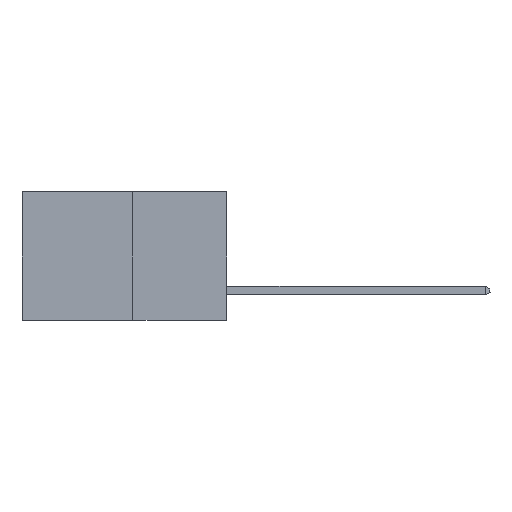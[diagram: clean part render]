
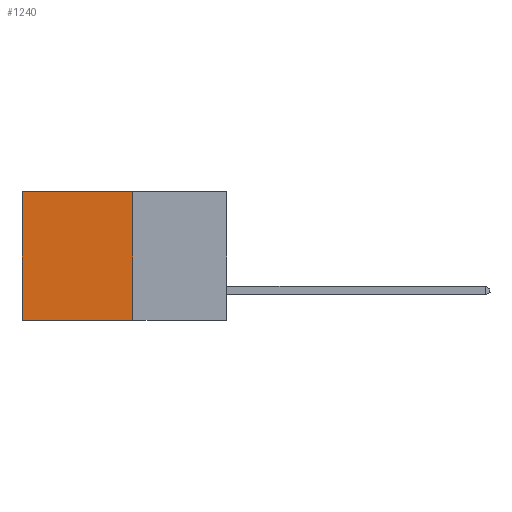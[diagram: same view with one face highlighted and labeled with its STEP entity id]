
A CAD part, left-side view. The second image highlights one B-rep face of the part: STEP entity #1240.
In plain terms, the highlighted planar face has unit normal (-1, 0, 0).
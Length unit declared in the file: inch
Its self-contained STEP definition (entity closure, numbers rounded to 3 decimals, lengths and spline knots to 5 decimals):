
#743 = CARTESIAN_POINT ( 'NONE',  ( 0.277, 0.59, -0.37 ) ) ;
#1240 = ADVANCED_FACE ( 'NONE', ( #14556 ), #4228, .F. ) ;
#2360 = LINE ( 'NONE', #743, #10150 ) ;
#2630 = CARTESIAN_POINT ( 'NONE',  ( 0.277, 0.27, 0. ) ) ;
#2664 = CARTESIAN_POINT ( 'NONE',  ( 0.277, 0.27, 0. ) ) ;
#2967 = ORIENTED_EDGE ( 'NONE', *, *, #3557, .F. ) ;
#3557 = EDGE_CURVE ( 'NONE', #14947, #12606, #7824, .T. ) ;
#4000 = ORIENTED_EDGE ( 'NONE', *, *, #9361, .T. ) ;
#4228 = PLANE ( 'NONE',  #18491 ) ;
#4608 = EDGE_LOOP ( 'NONE', ( #14594, #6383, #2967, #4000 ) ) ;
#4978 = CARTESIAN_POINT ( 'NONE',  ( 0.277, 0.27, -0.37 ) ) ;
#5147 = DIRECTION ( 'NONE',  ( 0., 0., -1. ) ) ;
#5317 = CARTESIAN_POINT ( 'NONE',  ( 0.277, 0.27, -0.37 ) ) ;
#6383 = ORIENTED_EDGE ( 'NONE', *, *, #18090, .F. ) ;
#6842 = CARTESIAN_POINT ( 'NONE',  ( 0.277, 0.59, -0.37 ) ) ;
#7334 = DIRECTION ( 'NONE',  ( 0., 0., -1. ) ) ;
#7824 = LINE ( 'NONE', #8733, #19585 ) ;
#7929 = DIRECTION ( 'NONE',  ( 1., 0., 0. ) ) ;
#8733 = CARTESIAN_POINT ( 'NONE',  ( 0.277, 0.27, -0.37 ) ) ;
#9361 = EDGE_CURVE ( 'NONE', #14947, #10341, #20909, .T. ) ;
#10150 = VECTOR ( 'NONE', #13995, 39.37008 ) ;
#10341 = VERTEX_POINT ( 'NONE', #10415 ) ;
#10415 = CARTESIAN_POINT ( 'NONE',  ( 0.277, 0.59, 0. ) ) ;
#12606 = VERTEX_POINT ( 'NONE', #14890 ) ;
#12668 = VERTEX_POINT ( 'NONE', #6842 ) ;
#13995 = DIRECTION ( 'NONE',  ( 0., 0., -1. ) ) ;
#14556 = FACE_OUTER_BOUND ( 'NONE', #4608, .T. ) ;
#14594 = ORIENTED_EDGE ( 'NONE', *, *, #16142, .T. ) ;
#14841 = DIRECTION ( 'NONE',  ( 0., 1., 0. ) ) ;
#14890 = CARTESIAN_POINT ( 'NONE',  ( 0.277, 0.27, -0.37 ) ) ;
#14947 = VERTEX_POINT ( 'NONE', #2630 ) ;
#15465 = VECTOR ( 'NONE', #14841, 39.37008 ) ;
#15926 = LINE ( 'NONE', #4978, #15465 ) ;
#16142 = EDGE_CURVE ( 'NONE', #10341, #12668, #2360, .T. ) ;
#16275 = VECTOR ( 'NONE', #18912, 39.37008 ) ;
#18090 = EDGE_CURVE ( 'NONE', #12606, #12668, #15926, .T. ) ;
#18491 = AXIS2_PLACEMENT_3D ( 'NONE', #5317, #7929, #5147 ) ;
#18912 = DIRECTION ( 'NONE',  ( 0., 1., 0. ) ) ;
#19585 = VECTOR ( 'NONE', #7334, 39.37008 ) ;
#20909 = LINE ( 'NONE', #2664, #16275 ) ;
